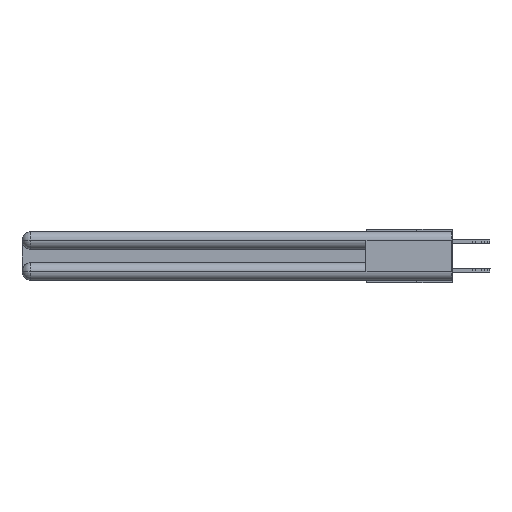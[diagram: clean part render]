
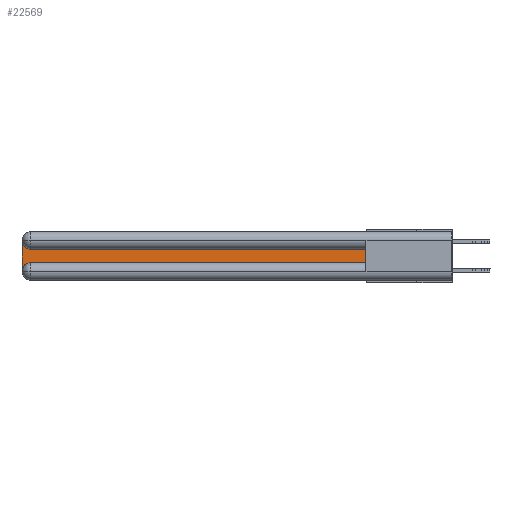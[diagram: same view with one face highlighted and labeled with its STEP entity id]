
A CAD part, left-side view. The second image highlights one B-rep face of the part: STEP entity #22569.
In plain terms, the highlighted planar face has unit normal (-1, 0, 0).
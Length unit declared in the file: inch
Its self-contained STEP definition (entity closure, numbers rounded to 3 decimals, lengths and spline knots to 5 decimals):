
#455 = CARTESIAN_POINT ( 'NONE',  ( 0.075, 0.6, -0.1225 ) ) ;
#569 = EDGE_CURVE ( 'NONE', #1125, #16408, #19310, .T. ) ;
#720 = CARTESIAN_POINT ( 'NONE',  ( 0.075, 0.6, -0.2175 ) ) ;
#772 = DIRECTION ( 'NONE',  ( 1., 0., 0. ) ) ;
#928 = ORIENTED_EDGE ( 'NONE', *, *, #25071, .T. ) ;
#1125 = VERTEX_POINT ( 'NONE', #24898 ) ;
#1386 = DIRECTION ( 'NONE',  ( 0., 0., -1. ) ) ;
#1754 = EDGE_CURVE ( 'NONE', #25447, #5801, #5901, .T. ) ;
#2576 = CARTESIAN_POINT ( 'NONE',  ( 0.075, 3., -0.2775 ) ) ;
#2613 = CIRCLE ( 'NONE', #2772, 0.06 ) ;
#2772 = AXIS2_PLACEMENT_3D ( 'NONE', #14597, #772, #7366 ) ;
#3117 = CARTESIAN_POINT ( 'NONE',  ( 0.075, 3., -0.1225 ) ) ;
#4814 = AXIS2_PLACEMENT_3D ( 'NONE', #10799, #20246, #1386 ) ;
#5801 = VERTEX_POINT ( 'NONE', #20777 ) ;
#5901 = LINE ( 'NONE', #9241, #28072 ) ;
#7162 = DIRECTION ( 'NONE',  ( 0., 1., 0. ) ) ;
#7366 = DIRECTION ( 'NONE',  ( 0., 0., -1. ) ) ;
#7895 = DIRECTION ( 'NONE',  ( 1., 0., 0. ) ) ;
#7926 = AXIS2_PLACEMENT_3D ( 'NONE', #3117, #7895, #17525 ) ;
#8979 = VECTOR ( 'NONE', #21160, 39.37008 ) ;
#9121 = ORIENTED_EDGE ( 'NONE', *, *, #29584, .T. ) ;
#9139 = ORIENTED_EDGE ( 'NONE', *, *, #16472, .T. ) ;
#9241 = CARTESIAN_POINT ( 'NONE',  ( 0.075, 0.6, -0.2175 ) ) ;
#9309 = CARTESIAN_POINT ( 'NONE',  ( 0.075, 2.94, -0.2175 ) ) ;
#10799 = CARTESIAN_POINT ( 'NONE',  ( 0.075, 2.94, -0.2775 ) ) ;
#11147 = VECTOR ( 'NONE', #7162, 39.37008 ) ;
#11763 = EDGE_LOOP ( 'NONE', ( #21971, #928, #9139, #9121, #25737, #24250 ) ) ;
#13529 = FACE_OUTER_BOUND ( 'NONE', #11763, .T. ) ;
#14597 = CARTESIAN_POINT ( 'NONE',  ( 0.075, 2.94, -0.0625 ) ) ;
#16408 = VERTEX_POINT ( 'NONE', #24403 ) ;
#16472 = EDGE_CURVE ( 'NONE', #21993, #19354, #23407, .T. ) ;
#17525 = DIRECTION ( 'NONE',  ( 0., 0., -1. ) ) ;
#19310 = LINE ( 'NONE', #455, #11147 ) ;
#19354 = VERTEX_POINT ( 'NONE', #2576 ) ;
#20137 = CIRCLE ( 'NONE', #4814, 0.06 ) ;
#20177 = DIRECTION ( 'NONE',  ( 0., 0., 1. ) ) ;
#20246 = DIRECTION ( 'NONE',  ( 1., 0., 0. ) ) ;
#20777 = CARTESIAN_POINT ( 'NONE',  ( 0.075, 0.6, -0.2175 ) ) ;
#21048 = DIRECTION ( 'NONE',  ( 0., -1., 0. ) ) ;
#21160 = DIRECTION ( 'NONE',  ( 0., 0., -1. ) ) ;
#21165 = CARTESIAN_POINT ( 'NONE',  ( 0.075, 3., -0.0625 ) ) ;
#21800 = EDGE_CURVE ( 'NONE', #5801, #1125, #25399, .T. ) ;
#21971 = ORIENTED_EDGE ( 'NONE', *, *, #569, .T. ) ;
#21993 = VERTEX_POINT ( 'NONE', #21165 ) ;
#22569 = ADVANCED_FACE ( 'NONE', ( #13529 ), #26897, .F. ) ;
#23407 = LINE ( 'NONE', #25863, #8979 ) ;
#24250 = ORIENTED_EDGE ( 'NONE', *, *, #21800, .T. ) ;
#24403 = CARTESIAN_POINT ( 'NONE',  ( 0.075, 2.94, -0.1225 ) ) ;
#24898 = CARTESIAN_POINT ( 'NONE',  ( 0.075, 0.6, -0.1225 ) ) ;
#25071 = EDGE_CURVE ( 'NONE', #16408, #21993, #2613, .T. ) ;
#25399 = LINE ( 'NONE', #720, #29128 ) ;
#25447 = VERTEX_POINT ( 'NONE', #9309 ) ;
#25737 = ORIENTED_EDGE ( 'NONE', *, *, #1754, .T. ) ;
#25863 = CARTESIAN_POINT ( 'NONE',  ( 0.075, 3., -0.2175 ) ) ;
#26897 = PLANE ( 'NONE',  #7926 ) ;
#28072 = VECTOR ( 'NONE', #21048, 39.37008 ) ;
#29128 = VECTOR ( 'NONE', #20177, 39.37008 ) ;
#29584 = EDGE_CURVE ( 'NONE', #19354, #25447, #20137, .T. ) ;
